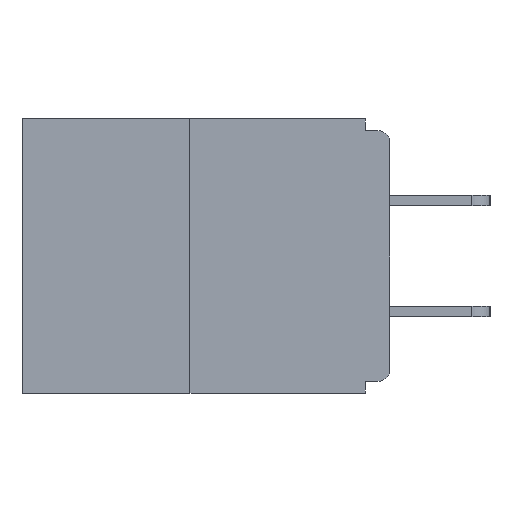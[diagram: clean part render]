
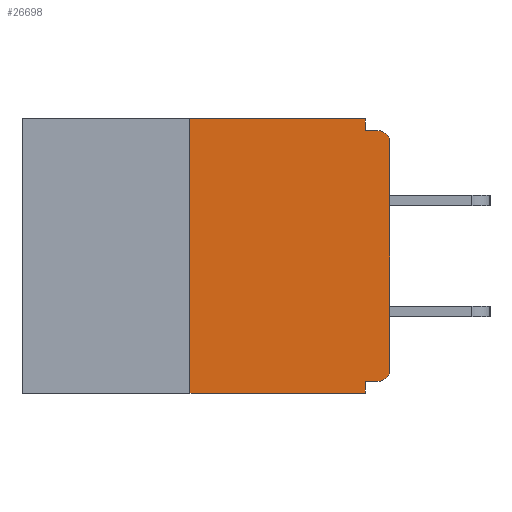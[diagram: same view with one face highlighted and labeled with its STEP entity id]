
A CAD part, left-side view. The second image highlights one B-rep face of the part: STEP entity #26698.
In plain terms, the highlighted planar face has unit normal (-1, 0, 0).
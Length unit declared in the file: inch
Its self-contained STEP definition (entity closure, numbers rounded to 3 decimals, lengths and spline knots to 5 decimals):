
#322 = EDGE_CURVE ( 'NONE', #22374, #18767, #2323, .T. ) ;
#394 = ORIENTED_EDGE ( 'NONE', *, *, #20049, .F. ) ;
#616 = CARTESIAN_POINT ( 'NONE',  ( 0., 0., -0.328 ) ) ;
#811 = CARTESIAN_POINT ( 'NONE',  ( 0., 0.015, -0.015 ) ) ;
#1256 = CARTESIAN_POINT ( 'NONE',  ( 0., 0.46, 0. ) ) ;
#1482 = LINE ( 'NONE', #19652, #16046 ) ;
#2271 = DIRECTION ( 'NONE',  ( 0., 0., -1. ) ) ;
#2323 = LINE ( 'NONE', #9612, #4882 ) ;
#3445 = CARTESIAN_POINT ( 'NONE',  ( 0., 0.031, 0. ) ) ;
#3653 = VERTEX_POINT ( 'NONE', #15636 ) ;
#3985 = EDGE_CURVE ( 'NONE', #10347, #7799, #10012, .T. ) ;
#4186 = EDGE_LOOP ( 'NONE', ( #17333, #26176, #9328, #27790, #7804, #29411, #25210, #28345, #17183, #394 ) ) ;
#4307 = CARTESIAN_POINT ( 'NONE',  ( 0., 0., -0.313 ) ) ;
#4323 = CARTESIAN_POINT ( 'NONE',  ( 0., 0.031, 0. ) ) ;
#4686 = VECTOR ( 'NONE', #2271, 39.37008 ) ;
#4882 = VECTOR ( 'NONE', #16465, 39.37008 ) ;
#4929 = CARTESIAN_POINT ( 'NONE',  ( 0., 0.031, -0.343 ) ) ;
#6087 = DIRECTION ( 'NONE',  ( 0., -1., 0. ) ) ;
#6403 = LINE ( 'NONE', #4323, #28722 ) ;
#6447 = CARTESIAN_POINT ( 'NONE',  ( 0., 0.031, -0.015 ) ) ;
#7151 = DIRECTION ( 'NONE',  ( -1., 0., 0. ) ) ;
#7182 = LINE ( 'NONE', #616, #17015 ) ;
#7338 = VECTOR ( 'NONE', #20842, 39.37008 ) ;
#7799 = VERTEX_POINT ( 'NONE', #811 ) ;
#7804 = ORIENTED_EDGE ( 'NONE', *, *, #17228, .F. ) ;
#8118 = DIRECTION ( 'NONE',  ( 1., 0., 0. ) ) ;
#8422 = AXIS2_PLACEMENT_3D ( 'NONE', #16393, #7151, #14001 ) ;
#8870 = VERTEX_POINT ( 'NONE', #3445 ) ;
#9128 = LINE ( 'NONE', #22659, #4686 ) ;
#9328 = ORIENTED_EDGE ( 'NONE', *, *, #14903, .T. ) ;
#9612 = CARTESIAN_POINT ( 'NONE',  ( 0., 0.25, 0. ) ) ;
#10012 = CIRCLE ( 'NONE', #19527, 0.015 ) ;
#10347 = VERTEX_POINT ( 'NONE', #16834 ) ;
#10519 = EDGE_CURVE ( 'NONE', #18767, #8870, #1482, .T. ) ;
#12187 = EDGE_CURVE ( 'NONE', #24158, #7799, #25461, .T. ) ;
#12437 = LINE ( 'NONE', #23576, #16586 ) ;
#14001 = DIRECTION ( 'NONE',  ( 0., 0., -1. ) ) ;
#14710 = DIRECTION ( 'NONE',  ( 0., 0., -1. ) ) ;
#14903 = EDGE_CURVE ( 'NONE', #22374, #17239, #16392, .T. ) ;
#14956 = DIRECTION ( 'NONE',  ( 0., 0., -1. ) ) ;
#15223 = VERTEX_POINT ( 'NONE', #4307 ) ;
#15636 = CARTESIAN_POINT ( 'NONE',  ( 0., 0.015, -0.328 ) ) ;
#16046 = VECTOR ( 'NONE', #6087, 39.37008 ) ;
#16392 = LINE ( 'NONE', #18921, #7338 ) ;
#16393 = CARTESIAN_POINT ( 'NONE',  ( 0., 0.015, -0.313 ) ) ;
#16465 = DIRECTION ( 'NONE',  ( 0., 0., 1. ) ) ;
#16586 = VECTOR ( 'NONE', #21802, 39.37008 ) ;
#16672 = CARTESIAN_POINT ( 'NONE',  ( 0., 0.015, -0.03 ) ) ;
#16834 = CARTESIAN_POINT ( 'NONE',  ( 0., 0., -0.03 ) ) ;
#17015 = VECTOR ( 'NONE', #18658, 39.37008 ) ;
#17183 = ORIENTED_EDGE ( 'NONE', *, *, #12187, .F. ) ;
#17228 = EDGE_CURVE ( 'NONE', #3653, #24799, #7182, .T. ) ;
#17239 = VERTEX_POINT ( 'NONE', #4929 ) ;
#17333 = ORIENTED_EDGE ( 'NONE', *, *, #10519, .F. ) ;
#18048 = VECTOR ( 'NONE', #18783, 39.37008 ) ;
#18658 = DIRECTION ( 'NONE',  ( 0., 1., 0. ) ) ;
#18691 = EDGE_CURVE ( 'NONE', #3653, #15223, #21247, .T. ) ;
#18767 = VERTEX_POINT ( 'NONE', #26214 ) ;
#18783 = DIRECTION ( 'NONE',  ( 0., -1., 0. ) ) ;
#18921 = CARTESIAN_POINT ( 'NONE',  ( 0., 0.46, -0.343 ) ) ;
#19527 = AXIS2_PLACEMENT_3D ( 'NONE', #16672, #28409, #14710 ) ;
#19591 = PLANE ( 'NONE',  #28427 ) ;
#19652 = CARTESIAN_POINT ( 'NONE',  ( 0., 0.46, 0. ) ) ;
#20049 = EDGE_CURVE ( 'NONE', #8870, #24158, #6403, .T. ) ;
#20842 = DIRECTION ( 'NONE',  ( 0., -1., 0. ) ) ;
#21004 = CARTESIAN_POINT ( 'NONE',  ( 0., 0., -0.015 ) ) ;
#21247 = CIRCLE ( 'NONE', #8422, 0.015 ) ;
#21644 = FACE_OUTER_BOUND ( 'NONE', #4186, .T. ) ;
#21802 = DIRECTION ( 'NONE',  ( 0., 0., 1. ) ) ;
#22330 = DIRECTION ( 'NONE',  ( 0., 0., -1. ) ) ;
#22374 = VERTEX_POINT ( 'NONE', #28102 ) ;
#22659 = CARTESIAN_POINT ( 'NONE',  ( 0., 0.031, -0.343 ) ) ;
#23576 = CARTESIAN_POINT ( 'NONE',  ( 0., 0., 0. ) ) ;
#23611 = CARTESIAN_POINT ( 'NONE',  ( 0., 0.031, -0.328 ) ) ;
#24158 = VERTEX_POINT ( 'NONE', #6447 ) ;
#24269 = EDGE_CURVE ( 'NONE', #24799, #17239, #9128, .T. ) ;
#24799 = VERTEX_POINT ( 'NONE', #23611 ) ;
#25210 = ORIENTED_EDGE ( 'NONE', *, *, #25254, .T. ) ;
#25254 = EDGE_CURVE ( 'NONE', #15223, #10347, #12437, .T. ) ;
#25461 = LINE ( 'NONE', #21004, #18048 ) ;
#26176 = ORIENTED_EDGE ( 'NONE', *, *, #322, .F. ) ;
#26214 = CARTESIAN_POINT ( 'NONE',  ( 0., 0.25, 0. ) ) ;
#26698 = ADVANCED_FACE ( 'NONE', ( #21644 ), #19591, .F. ) ;
#27790 = ORIENTED_EDGE ( 'NONE', *, *, #24269, .F. ) ;
#28102 = CARTESIAN_POINT ( 'NONE',  ( 0., 0.25, -0.343 ) ) ;
#28345 = ORIENTED_EDGE ( 'NONE', *, *, #3985, .T. ) ;
#28409 = DIRECTION ( 'NONE',  ( -1., 0., 0. ) ) ;
#28427 = AXIS2_PLACEMENT_3D ( 'NONE', #1256, #8118, #14956 ) ;
#28722 = VECTOR ( 'NONE', #22330, 39.37008 ) ;
#29411 = ORIENTED_EDGE ( 'NONE', *, *, #18691, .T. ) ;
